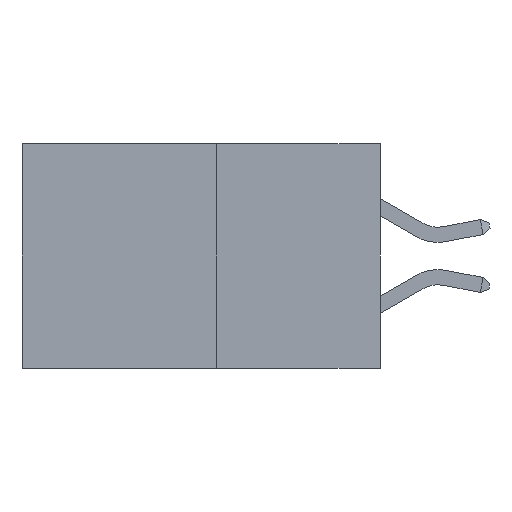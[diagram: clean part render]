
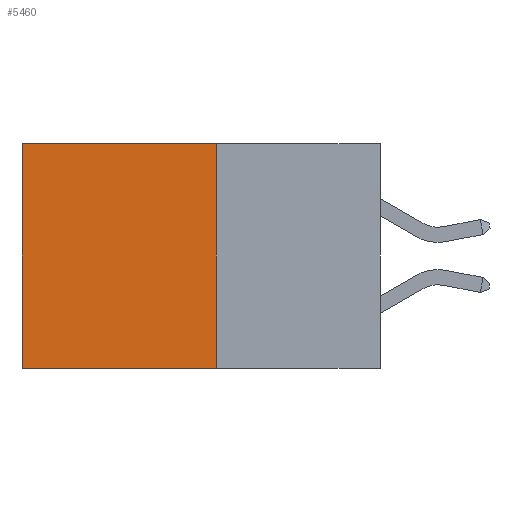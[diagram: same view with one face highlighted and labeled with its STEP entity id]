
A CAD part, left-side view. The second image highlights one B-rep face of the part: STEP entity #5460.
In plain terms, the highlighted planar face has unit normal (-1, 0, 0).
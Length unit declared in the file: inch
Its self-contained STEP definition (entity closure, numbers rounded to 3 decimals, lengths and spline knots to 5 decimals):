
#167 = DIRECTION ( 'NONE',  ( 0., 0., -1. ) ) ;
#330 = VERTEX_POINT ( 'NONE', #11242 ) ;
#393 = CARTESIAN_POINT ( 'NONE',  ( 0.277, 0.27, -0.37 ) ) ;
#496 = EDGE_LOOP ( 'NONE', ( #6354, #6686, #12090, #6878 ) ) ;
#1339 = CARTESIAN_POINT ( 'NONE',  ( 0.277, 0.27, 0. ) ) ;
#1723 = CARTESIAN_POINT ( 'NONE',  ( 0.277, 0.27, 0. ) ) ;
#2077 = VECTOR ( 'NONE', #2410, 39.37008 ) ;
#2410 = DIRECTION ( 'NONE',  ( 0., 1., 0. ) ) ;
#2598 = VERTEX_POINT ( 'NONE', #7654 ) ;
#2725 = VECTOR ( 'NONE', #12003, 39.37008 ) ;
#3299 = AXIS2_PLACEMENT_3D ( 'NONE', #4445, #9651, #3433 ) ;
#3433 = DIRECTION ( 'NONE',  ( 0., 0., -1. ) ) ;
#3882 = LINE ( 'NONE', #7522, #6353 ) ;
#4445 = CARTESIAN_POINT ( 'NONE',  ( 0.277, 0.27, -0.37 ) ) ;
#4518 = VERTEX_POINT ( 'NONE', #1723 ) ;
#5460 = ADVANCED_FACE ( 'NONE', ( #10042 ), #8629, .F. ) ;
#5488 = EDGE_CURVE ( 'NONE', #4518, #330, #7341, .T. ) ;
#5543 = VECTOR ( 'NONE', #11118, 39.37008 ) ;
#6017 = EDGE_CURVE ( 'NONE', #330, #2598, #3882, .T. ) ;
#6185 = VERTEX_POINT ( 'NONE', #393 ) ;
#6306 = EDGE_CURVE ( 'NONE', #4518, #6185, #8610, .T. ) ;
#6353 = VECTOR ( 'NONE', #167, 39.37008 ) ;
#6354 = ORIENTED_EDGE ( 'NONE', *, *, #6017, .T. ) ;
#6686 = ORIENTED_EDGE ( 'NONE', *, *, #10141, .F. ) ;
#6878 = ORIENTED_EDGE ( 'NONE', *, *, #5488, .T. ) ;
#7023 = CARTESIAN_POINT ( 'NONE',  ( 0.277, 0.27, -0.37 ) ) ;
#7341 = LINE ( 'NONE', #1339, #2077 ) ;
#7522 = CARTESIAN_POINT ( 'NONE',  ( 0.277, 0.59, -0.37 ) ) ;
#7654 = CARTESIAN_POINT ( 'NONE',  ( 0.277, 0.59, -0.37 ) ) ;
#8610 = LINE ( 'NONE', #9946, #2725 ) ;
#8629 = PLANE ( 'NONE',  #3299 ) ;
#9651 = DIRECTION ( 'NONE',  ( 1., 0., 0. ) ) ;
#9946 = CARTESIAN_POINT ( 'NONE',  ( 0.277, 0.27, -0.37 ) ) ;
#10042 = FACE_OUTER_BOUND ( 'NONE', #496, .T. ) ;
#10141 = EDGE_CURVE ( 'NONE', #6185, #2598, #11380, .T. ) ;
#11118 = DIRECTION ( 'NONE',  ( 0., 1., 0. ) ) ;
#11242 = CARTESIAN_POINT ( 'NONE',  ( 0.277, 0.59, 0. ) ) ;
#11380 = LINE ( 'NONE', #7023, #5543 ) ;
#12003 = DIRECTION ( 'NONE',  ( 0., 0., -1. ) ) ;
#12090 = ORIENTED_EDGE ( 'NONE', *, *, #6306, .F. ) ;
